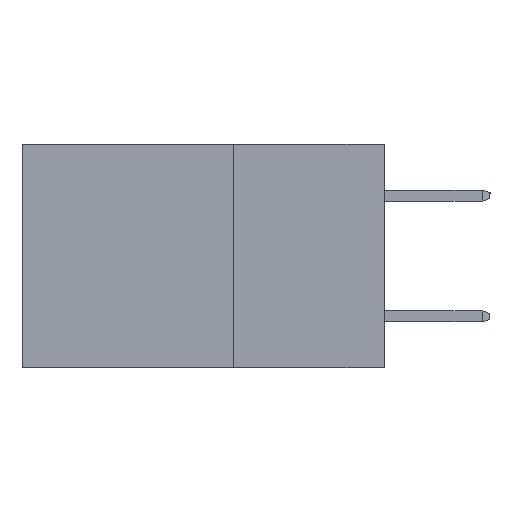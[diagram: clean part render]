
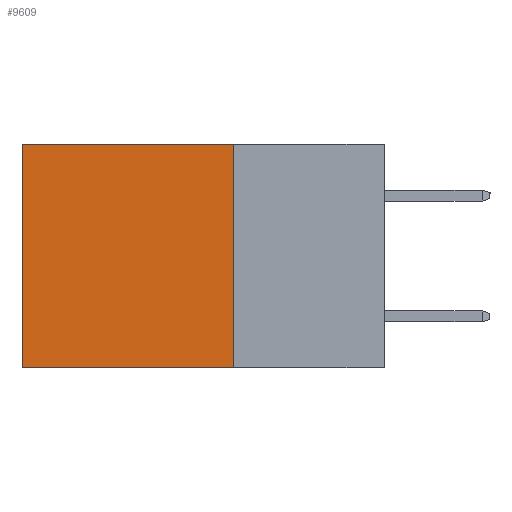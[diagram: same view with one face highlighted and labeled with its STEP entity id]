
A CAD part, left-side view. The second image highlights one B-rep face of the part: STEP entity #9609.
In plain terms, the highlighted planar face has unit normal (-1, 0, 0).
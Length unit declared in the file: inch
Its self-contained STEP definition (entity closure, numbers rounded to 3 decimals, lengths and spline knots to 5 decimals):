
#177 = LINE ( 'NONE', #11207, #4129 ) ;
#237 = AXIS2_PLACEMENT_3D ( 'NONE', #7411, #4272, #3418 ) ;
#433 = EDGE_CURVE ( 'NONE', #9398, #4042, #6657, .T. ) ;
#1120 = VERTEX_POINT ( 'NONE', #9265 ) ;
#1311 = CARTESIAN_POINT ( 'NONE',  ( 0.2615, 0.25, 0. ) ) ;
#1387 = EDGE_CURVE ( 'NONE', #1120, #12248, #4626, .T. ) ;
#1753 = CARTESIAN_POINT ( 'NONE',  ( 0.2615, 0.25, -0.37 ) ) ;
#2273 = PLANE ( 'NONE',  #237 ) ;
#2394 = FACE_OUTER_BOUND ( 'NONE', #11142, .T. ) ;
#2539 = DIRECTION ( 'NONE',  ( 0., 0., -1. ) ) ;
#3418 = DIRECTION ( 'NONE',  ( 0., 0., -1. ) ) ;
#4042 = VERTEX_POINT ( 'NONE', #5756 ) ;
#4129 = VECTOR ( 'NONE', #10207, 39.37008 ) ;
#4272 = DIRECTION ( 'NONE',  ( 1., 0., 0. ) ) ;
#4563 = ORIENTED_EDGE ( 'NONE', *, *, #1387, .F. ) ;
#4626 = LINE ( 'NONE', #9797, #5897 ) ;
#5134 = EDGE_CURVE ( 'NONE', #12248, #4042, #177, .T. ) ;
#5416 = ORIENTED_EDGE ( 'NONE', *, *, #5134, .F. ) ;
#5475 = VECTOR ( 'NONE', #2539, 39.37008 ) ;
#5756 = CARTESIAN_POINT ( 'NONE',  ( 0.2615, 0.6, -0.37 ) ) ;
#5877 = ORIENTED_EDGE ( 'NONE', *, *, #9649, .T. ) ;
#5897 = VECTOR ( 'NONE', #6993, 39.37008 ) ;
#6582 = CARTESIAN_POINT ( 'NONE',  ( 0.2615, 0.6, -0.37 ) ) ;
#6657 = LINE ( 'NONE', #6582, #5475 ) ;
#6993 = DIRECTION ( 'NONE',  ( 0., 0., -1. ) ) ;
#7229 = CARTESIAN_POINT ( 'NONE',  ( 0.2615, 0.6, 0. ) ) ;
#7411 = CARTESIAN_POINT ( 'NONE',  ( 0.2615, 0.25, -0.37 ) ) ;
#7799 = VECTOR ( 'NONE', #10363, 39.37008 ) ;
#9265 = CARTESIAN_POINT ( 'NONE',  ( 0.2615, 0.25, 0. ) ) ;
#9398 = VERTEX_POINT ( 'NONE', #7229 ) ;
#9435 = LINE ( 'NONE', #1311, #7799 ) ;
#9609 = ADVANCED_FACE ( 'NONE', ( #2394 ), #2273, .F. ) ;
#9649 = EDGE_CURVE ( 'NONE', #1120, #9398, #9435, .T. ) ;
#9797 = CARTESIAN_POINT ( 'NONE',  ( 0.2615, 0.25, -0.37 ) ) ;
#10207 = DIRECTION ( 'NONE',  ( 0., 1., 0. ) ) ;
#10363 = DIRECTION ( 'NONE',  ( 0., 1., 0. ) ) ;
#11142 = EDGE_LOOP ( 'NONE', ( #12516, #5416, #4563, #5877 ) ) ;
#11207 = CARTESIAN_POINT ( 'NONE',  ( 0.2615, 0.25, -0.37 ) ) ;
#12248 = VERTEX_POINT ( 'NONE', #1753 ) ;
#12516 = ORIENTED_EDGE ( 'NONE', *, *, #433, .T. ) ;
